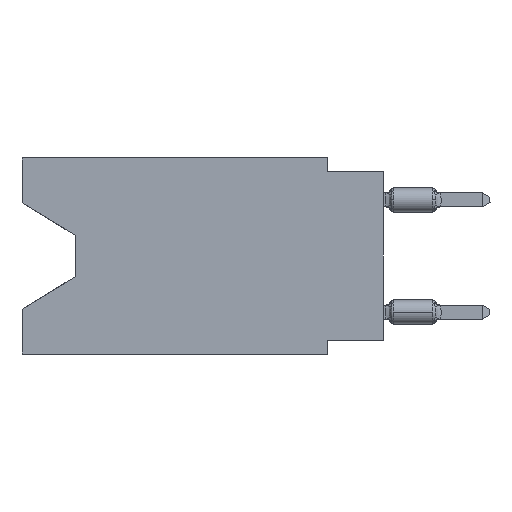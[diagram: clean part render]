
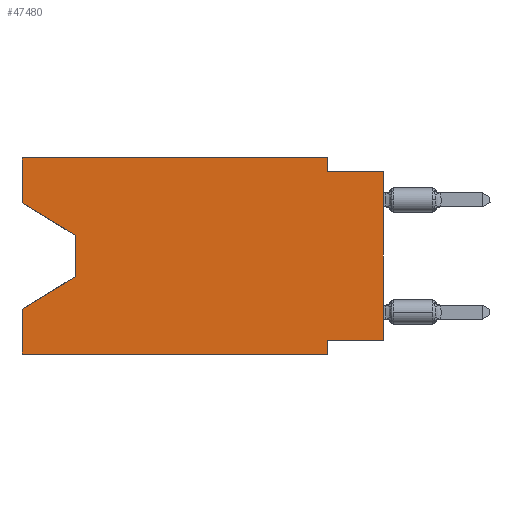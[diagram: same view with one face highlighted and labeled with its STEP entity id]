
A CAD part, left-side view. The second image highlights one B-rep face of the part: STEP entity #47480.
In plain terms, the highlighted planar face has unit normal (-1, 0, 0).
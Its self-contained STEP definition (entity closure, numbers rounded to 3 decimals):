
#184 = CARTESIAN_POINT ( 'NONE',  ( 0., 0., -8.255 ) ) ;
#673 = CARTESIAN_POINT ( 'NONE',  ( 0., 13.97, -5.385 ) ) ;
#702 = LINE ( 'NONE', #15617, #39164 ) ;
#4059 = CARTESIAN_POINT ( 'NONE',  ( 0., 13.97, -5.385 ) ) ;
#4094 = CARTESIAN_POINT ( 'NONE',  ( 0., 2.54, 0. ) ) ;
#5146 = DIRECTION ( 'NONE',  ( 0., 0., -1. ) ) ;
#5172 = VECTOR ( 'NONE', #61865, 1000. ) ;
#5176 = AXIS2_PLACEMENT_3D ( 'NONE', #48306, #38197, #48013 ) ;
#5318 = EDGE_CURVE ( 'NONE', #31225, #59896, #28322, .T. ) ;
#8745 = FACE_OUTER_BOUND ( 'NONE', #17908, .T. ) ;
#9169 = CARTESIAN_POINT ( 'NONE',  ( 0., 16.383, 0. ) ) ;
#9218 = CARTESIAN_POINT ( 'NONE',  ( 0., 2.54, -8.89 ) ) ;
#9259 = DIRECTION ( 'NONE',  ( 0., 0., 1. ) ) ;
#9872 = VERTEX_POINT ( 'NONE', #58630 ) ;
#10846 = VECTOR ( 'NONE', #9259, 1000. ) ;
#11543 = LINE ( 'NONE', #58377, #33488 ) ;
#12124 = EDGE_CURVE ( 'NONE', #9872, #13458, #28202, .T. ) ;
#12808 = CARTESIAN_POINT ( 'NONE',  ( 0., 0., -0.635 ) ) ;
#12984 = CARTESIAN_POINT ( 'NONE',  ( 0., 13.97, -3.505 ) ) ;
#13168 = CARTESIAN_POINT ( 'NONE',  ( 0., 16.383, -2.038 ) ) ;
#13431 = DIRECTION ( 'NONE',  ( 0., -1., 0. ) ) ;
#13458 = VERTEX_POINT ( 'NONE', #26777 ) ;
#13825 = CARTESIAN_POINT ( 'NONE',  ( 0., 16.383, 0. ) ) ;
#14164 = EDGE_CURVE ( 'NONE', #19668, #30465, #11543, .T. ) ;
#14384 = ORIENTED_EDGE ( 'NONE', *, *, #21980, .F. ) ;
#14952 = VERTEX_POINT ( 'NONE', #4094 ) ;
#15068 = CARTESIAN_POINT ( 'NONE',  ( 0., 0., -8.255 ) ) ;
#15617 = CARTESIAN_POINT ( 'NONE',  ( 0., 13.97, -3.505 ) ) ;
#15736 = VECTOR ( 'NONE', #5146, 1000. ) ;
#15967 = DIRECTION ( 'NONE',  ( 0., 0., -1. ) ) ;
#17423 = EDGE_CURVE ( 'NONE', #9872, #30465, #22459, .T. ) ;
#17465 = CARTESIAN_POINT ( 'NONE',  ( 0., 0., -0.635 ) ) ;
#17908 = EDGE_LOOP ( 'NONE', ( #33820, #53055, #44518, #19413, #18903, #45434, #30010, #51087, #40406, #59237, #14384, #52111 ) ) ;
#18903 = ORIENTED_EDGE ( 'NONE', *, *, #17423, .T. ) ;
#19413 = ORIENTED_EDGE ( 'NONE', *, *, #12124, .F. ) ;
#19668 = VERTEX_POINT ( 'NONE', #29448 ) ;
#20105 = EDGE_CURVE ( 'NONE', #61573, #24162, #702, .T. ) ;
#21980 = EDGE_CURVE ( 'NONE', #25884, #14952, #29045, .T. ) ;
#22274 = VECTOR ( 'NONE', #24297, 1000. ) ;
#22459 = LINE ( 'NONE', #41436, #25297 ) ;
#24162 = VERTEX_POINT ( 'NONE', #4059 ) ;
#24297 = DIRECTION ( 'NONE',  ( 0., -1., 0. ) ) ;
#24419 = VECTOR ( 'NONE', #47185, 1000. ) ;
#25120 = CARTESIAN_POINT ( 'NONE',  ( 0., 2.54, 0. ) ) ;
#25297 = VECTOR ( 'NONE', #51862, 1000. ) ;
#25368 = CARTESIAN_POINT ( 'NONE',  ( 0., 16.383, -2.038 ) ) ;
#25884 = VERTEX_POINT ( 'NONE', #54771 ) ;
#26777 = CARTESIAN_POINT ( 'NONE',  ( 0., 16.383, -6.852 ) ) ;
#28172 = VECTOR ( 'NONE', #31696, 1000. ) ;
#28202 = LINE ( 'NONE', #9169, #24419 ) ;
#28322 = LINE ( 'NONE', #52059, #5172 ) ;
#28615 = CARTESIAN_POINT ( 'NONE',  ( 0., 16.383, 0. ) ) ;
#28729 = PLANE ( 'NONE',  #5176 ) ;
#28896 = EDGE_CURVE ( 'NONE', #14952, #62249, #48524, .T. ) ;
#29045 = LINE ( 'NONE', #13825, #22274 ) ;
#29448 = CARTESIAN_POINT ( 'NONE',  ( 0., 2.54, -8.255 ) ) ;
#30010 = ORIENTED_EDGE ( 'NONE', *, *, #57555, .F. ) ;
#30120 = LINE ( 'NONE', #25368, #28172 ) ;
#30465 = VERTEX_POINT ( 'NONE', #9218 ) ;
#31225 = VERTEX_POINT ( 'NONE', #184 ) ;
#31696 = DIRECTION ( 'NONE',  ( 0., -0.855, -0.519 ) ) ;
#33317 = VERTEX_POINT ( 'NONE', #13168 ) ;
#33329 = LINE ( 'NONE', #28615, #10846 ) ;
#33488 = VECTOR ( 'NONE', #15967, 1000. ) ;
#33820 = ORIENTED_EDGE ( 'NONE', *, *, #36962, .T. ) ;
#36962 = EDGE_CURVE ( 'NONE', #33317, #61573, #30120, .T. ) ;
#38197 = DIRECTION ( 'NONE',  ( 1., 0., 0. ) ) ;
#39164 = VECTOR ( 'NONE', #49156, 1000. ) ;
#39644 = DIRECTION ( 'NONE',  ( 0., 0.855, -0.519 ) ) ;
#40406 = ORIENTED_EDGE ( 'NONE', *, *, #54089, .F. ) ;
#41436 = CARTESIAN_POINT ( 'NONE',  ( 0., 16.383, -8.89 ) ) ;
#42248 = LINE ( 'NONE', #12808, #48786 ) ;
#43533 = CARTESIAN_POINT ( 'NONE',  ( 0., 2.54, -0.635 ) ) ;
#44518 = ORIENTED_EDGE ( 'NONE', *, *, #57050, .T. ) ;
#45434 = ORIENTED_EDGE ( 'NONE', *, *, #14164, .F. ) ;
#47055 = VECTOR ( 'NONE', #59077, 1000. ) ;
#47185 = DIRECTION ( 'NONE',  ( 0., 0., 1. ) ) ;
#47480 = ADVANCED_FACE ( 'NONE', ( #8745 ), #28729, .F. ) ;
#48013 = DIRECTION ( 'NONE',  ( 0., 0., -1. ) ) ;
#48306 = CARTESIAN_POINT ( 'NONE',  ( 0., 16.383, 0. ) ) ;
#48488 = LINE ( 'NONE', #673, #55126 ) ;
#48524 = LINE ( 'NONE', #25120, #15736 ) ;
#48786 = VECTOR ( 'NONE', #13431, 1000. ) ;
#49156 = DIRECTION ( 'NONE',  ( 0., 0., -1. ) ) ;
#51087 = ORIENTED_EDGE ( 'NONE', *, *, #5318, .T. ) ;
#51862 = DIRECTION ( 'NONE',  ( 0., -1., 0. ) ) ;
#52059 = CARTESIAN_POINT ( 'NONE',  ( 0., 0., 0. ) ) ;
#52111 = ORIENTED_EDGE ( 'NONE', *, *, #61433, .F. ) ;
#53055 = ORIENTED_EDGE ( 'NONE', *, *, #20105, .T. ) ;
#54089 = EDGE_CURVE ( 'NONE', #62249, #59896, #42248, .T. ) ;
#54771 = CARTESIAN_POINT ( 'NONE',  ( 0., 16.383, 0. ) ) ;
#55126 = VECTOR ( 'NONE', #39644, 1000. ) ;
#57050 = EDGE_CURVE ( 'NONE', #24162, #13458, #48488, .T. ) ;
#57555 = EDGE_CURVE ( 'NONE', #31225, #19668, #58426, .T. ) ;
#58377 = CARTESIAN_POINT ( 'NONE',  ( 0., 2.54, -8.89 ) ) ;
#58426 = LINE ( 'NONE', #15068, #47055 ) ;
#58630 = CARTESIAN_POINT ( 'NONE',  ( 0., 16.383, -8.89 ) ) ;
#59077 = DIRECTION ( 'NONE',  ( 0., 1., 0. ) ) ;
#59237 = ORIENTED_EDGE ( 'NONE', *, *, #28896, .F. ) ;
#59896 = VERTEX_POINT ( 'NONE', #17465 ) ;
#61433 = EDGE_CURVE ( 'NONE', #33317, #25884, #33329, .T. ) ;
#61573 = VERTEX_POINT ( 'NONE', #12984 ) ;
#61865 = DIRECTION ( 'NONE',  ( 0., 0., 1. ) ) ;
#62249 = VERTEX_POINT ( 'NONE', #43533 ) ;
